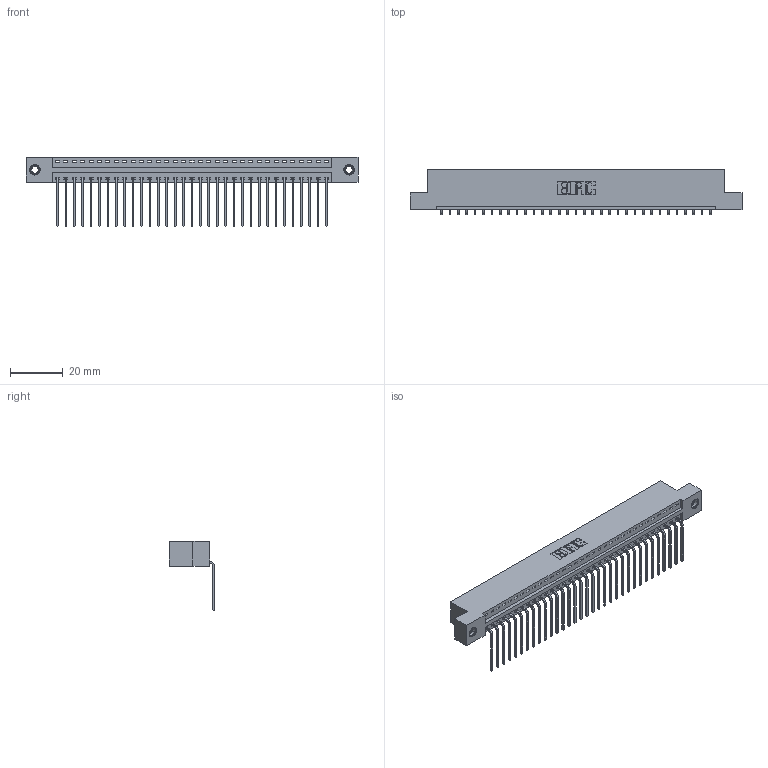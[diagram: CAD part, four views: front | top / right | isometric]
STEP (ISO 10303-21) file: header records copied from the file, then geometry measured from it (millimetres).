
FILE_DESCRIPTION (( 'STEP AP203' ), '1' );
FILE_NAME ('396-033-559-107.STEP', '2018-09-05T23:40:06', ( '' ), ( '' ), 'SwSTEP 2.0', 'SolidWorks 2016', '' );
FILE_SCHEMA (( 'CONFIG_CONTROL_DESIGN' ));
Length unit declared in the file: inch
Products named in the file (4): 346 Part_Flush Mounting Lugs - 0.156 Dia-TI; 345-292-001_558 559 Tail - 1; 345-250-001_345-250-005-103; 396-033-559-107
Assembly tree (36 placements, depth 2):
  396-033-559-107
    346 Part_Flush Mounting Lugs - 0.156 Dia-TI
    345-292-001_558 559 Tail - 1  x33
    345-250-001_345-250-005-103  x2
Bounding box: 125.35 x 17.08 x 26.16 mm (x, y, z)
Volume: 12033.1 mm3; surface area: 15633.3 mm2
Topology: 36 solids, 36 shells, 2162 faces, 6471 edges, 4262 vertices
Faces by surface type: plane 1494, cylinder 652, cone 12, torus 4
Entity records: 22962 total; most frequent: CARTESIAN_POINT 3922, ORIENTED_EDGE 3882, DIRECTION 3497, EDGE_CURVE 1941, VECTOR 1657, LINE 1657, VERTEX_POINT 1288, AXIS2_PLACEMENT_3D 920
